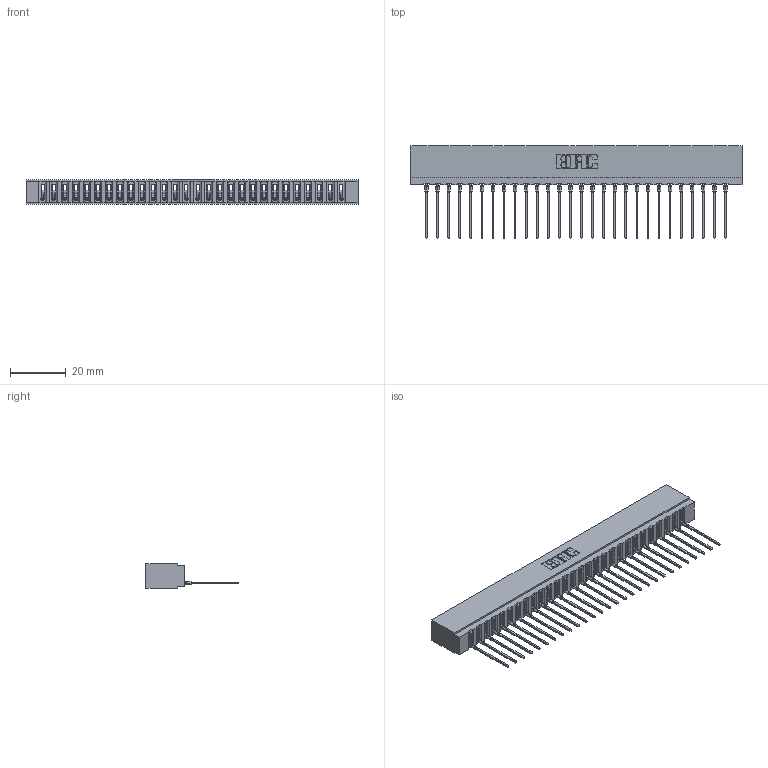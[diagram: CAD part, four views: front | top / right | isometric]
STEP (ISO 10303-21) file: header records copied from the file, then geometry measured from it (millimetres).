
FILE_DESCRIPTION (( 'STEP AP203' ), '1' );
FILE_NAME ('717-028-541-101.STEP', '2026-02-20T21:15:27', ( '' ), ( '' ), 'SwSTEP 2.0', 'SolidWorks 2023', '' );
FILE_SCHEMA (( 'CONFIG_CONTROL_DESIGN' ));
Length unit declared in the file: millimetre
Products named in the file (3): 717 Part_Insulator Option - 06; 717-028-541-101; 745-292-001_541
Assembly tree (29 placements, depth 2):
  717-028-541-101
    717 Part_Insulator Option - 06
    745-292-001_541  x28
Bounding box: 118.82 x 33.01 x 8.89 mm (x, y, z)
Volume: 10216.4 mm3; surface area: 14788 mm2
Topology: 29 solids, 29 shells, 3258 faces, 8959 edges, 5654 vertices
Faces by surface type: plane 1958, cylinder 572, bspline 560, torus 168
Entity records: 49009 total; most frequent: CARTESIAN_POINT 9141, ORIENTED_EDGE 8576, DIRECTION 7444, EDGE_CURVE 4288, VECTOR 3938, LINE 3938, VERTEX_POINT 2738, AXIS2_PLACEMENT_3D 1753
